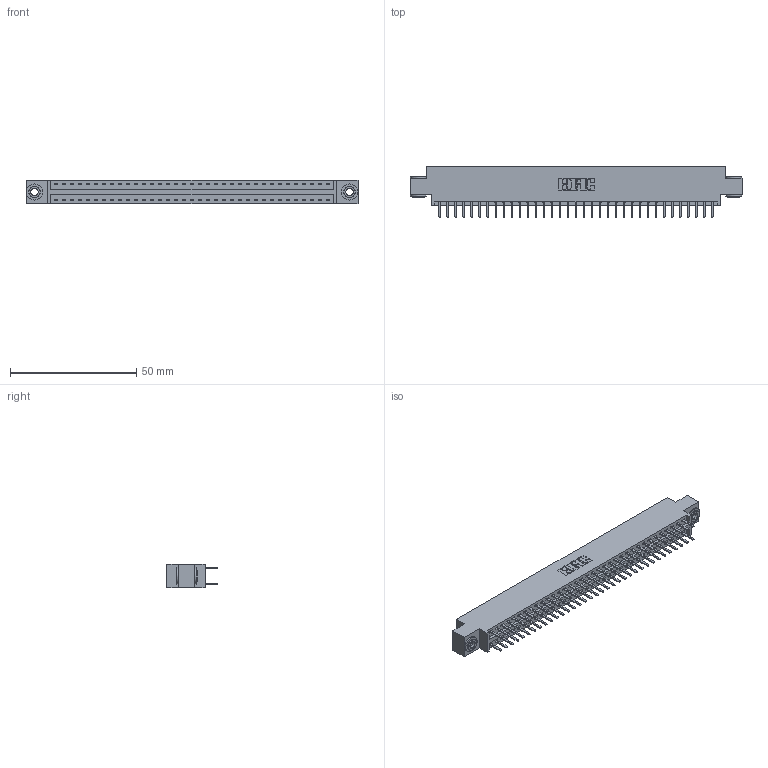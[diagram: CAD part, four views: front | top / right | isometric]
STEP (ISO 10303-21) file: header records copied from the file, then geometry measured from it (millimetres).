
FILE_DESCRIPTION (( 'STEP AP203' ), '1' );
FILE_NAME ('346-070-520-803.STEP', '2022-05-24T20:48:52', ( '' ), ( '' ), 'SwSTEP 2.0', 'SolidWorks 2020', '' );
FILE_SCHEMA (( 'CONFIG_CONTROL_DESIGN' ));
Length unit declared in the file: inch
Products named in the file (4): 346-070-520-803; 345-292-001_345-293-120; 345-250-002_345-250-002-102; 346 Part_0.170 Offset - 0.156 Dia-TH
Assembly tree (73 placements, depth 2):
  346-070-520-803
    346 Part_0.170 Offset - 0.156 Dia-TH
    345-292-001_345-293-120  x70
    345-250-002_345-250-002-102  x2
Bounding box: 131.7 x 20.02 x 9.4 mm (x, y, z)
Volume: 12603.8 mm3; surface area: 17571 mm2
Topology: 73 solids, 73 shells, 4098 faces, 11863 edges, 7718 vertices
Faces by surface type: plane 2694, cylinder 1396, cone 8
Entity records: 25096 total; most frequent: CARTESIAN_POINT 4141, ORIENTED_EDGE 4054, DIRECTION 3717, EDGE_CURVE 2027, VECTOR 1727, LINE 1727, VERTEX_POINT 1346, AXIS2_PLACEMENT_3D 995
